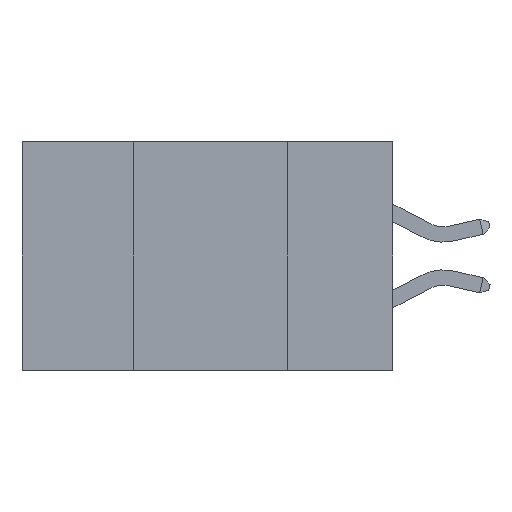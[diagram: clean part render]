
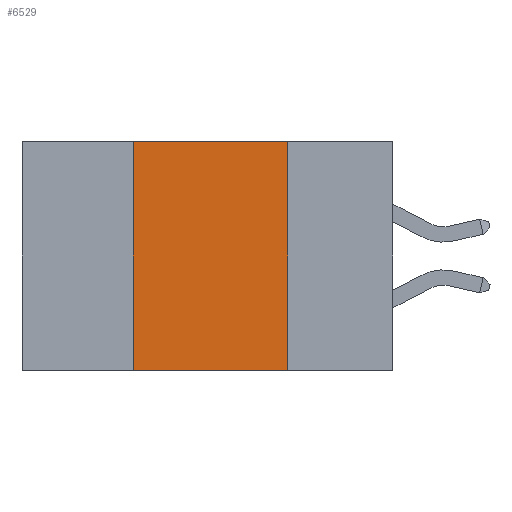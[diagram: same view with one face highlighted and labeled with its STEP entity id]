
A CAD part, left-side view. The second image highlights one B-rep face of the part: STEP entity #6529.
In plain terms, the highlighted planar face has unit normal (-1, 0, 0).
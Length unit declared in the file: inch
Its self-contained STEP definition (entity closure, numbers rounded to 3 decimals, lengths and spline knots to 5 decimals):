
#419 = DIRECTION ( 'NONE',  ( 0., 0., -1. ) ) ;
#474 = ORIENTED_EDGE ( 'NONE', *, *, #3820, .T. ) ;
#1090 = AXIS2_PLACEMENT_3D ( 'NONE', #14772, #7922, #17565 ) ;
#1649 = CARTESIAN_POINT ( 'NONE',  ( 0., 0.42, -0.37 ) ) ;
#2009 = VECTOR ( 'NONE', #419, 39.37008 ) ;
#3423 = EDGE_CURVE ( 'NONE', #3634, #11902, #14747, .T. ) ;
#3570 = VECTOR ( 'NONE', #7250, 39.37008 ) ;
#3634 = VERTEX_POINT ( 'NONE', #14753 ) ;
#3820 = EDGE_CURVE ( 'NONE', #10285, #15336, #13870, .T. ) ;
#4199 = CARTESIAN_POINT ( 'NONE',  ( 0., 0.6, -0.37 ) ) ;
#4299 = CARTESIAN_POINT ( 'NONE',  ( 0., 0.6, 0. ) ) ;
#4952 = CARTESIAN_POINT ( 'NONE',  ( 0., 0.17, 0. ) ) ;
#5188 = EDGE_CURVE ( 'NONE', #11902, #15336, #13366, .T. ) ;
#6529 = ADVANCED_FACE ( 'NONE', ( #8154 ), #13394, .F. ) ;
#7250 = DIRECTION ( 'NONE',  ( 0., -1., 0. ) ) ;
#7922 = DIRECTION ( 'NONE',  ( 1., 0., 0. ) ) ;
#8154 = FACE_OUTER_BOUND ( 'NONE', #14036, .T. ) ;
#8311 = CARTESIAN_POINT ( 'NONE',  ( 0., 0.17, 0. ) ) ;
#8475 = DIRECTION ( 'NONE',  ( 0., -1., 0. ) ) ;
#9363 = VECTOR ( 'NONE', #17748, 39.37008 ) ;
#9755 = VECTOR ( 'NONE', #8475, 39.37008 ) ;
#9792 = CARTESIAN_POINT ( 'NONE',  ( 0., 0.17, -0.37 ) ) ;
#10285 = VERTEX_POINT ( 'NONE', #1649 ) ;
#10774 = EDGE_CURVE ( 'NONE', #10285, #3634, #16705, .T. ) ;
#11902 = VERTEX_POINT ( 'NONE', #8311 ) ;
#13366 = LINE ( 'NONE', #4952, #2009 ) ;
#13394 = PLANE ( 'NONE',  #1090 ) ;
#13870 = LINE ( 'NONE', #4199, #9755 ) ;
#14036 = EDGE_LOOP ( 'NONE', ( #14122, #14314, #15240, #474 ) ) ;
#14122 = ORIENTED_EDGE ( 'NONE', *, *, #5188, .F. ) ;
#14314 = ORIENTED_EDGE ( 'NONE', *, *, #3423, .F. ) ;
#14747 = LINE ( 'NONE', #4299, #3570 ) ;
#14753 = CARTESIAN_POINT ( 'NONE',  ( 0., 0.42, 0. ) ) ;
#14772 = CARTESIAN_POINT ( 'NONE',  ( 0., 0.6, 0. ) ) ;
#15240 = ORIENTED_EDGE ( 'NONE', *, *, #10774, .F. ) ;
#15336 = VERTEX_POINT ( 'NONE', #9792 ) ;
#16364 = CARTESIAN_POINT ( 'NONE',  ( 0., 0.42, 0. ) ) ;
#16705 = LINE ( 'NONE', #16364, #9363 ) ;
#17565 = DIRECTION ( 'NONE',  ( 0., 0., -1. ) ) ;
#17748 = DIRECTION ( 'NONE',  ( 0., 0., 1. ) ) ;
